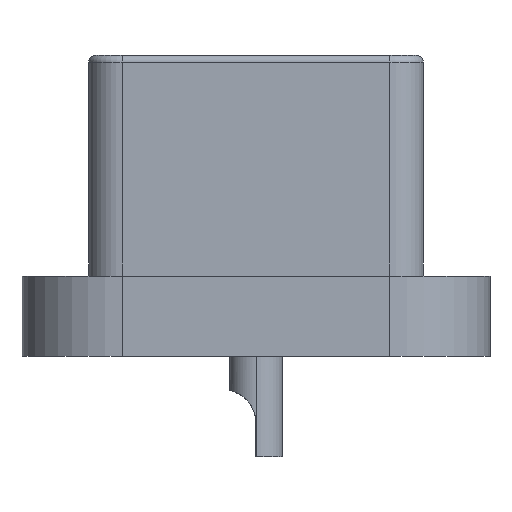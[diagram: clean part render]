
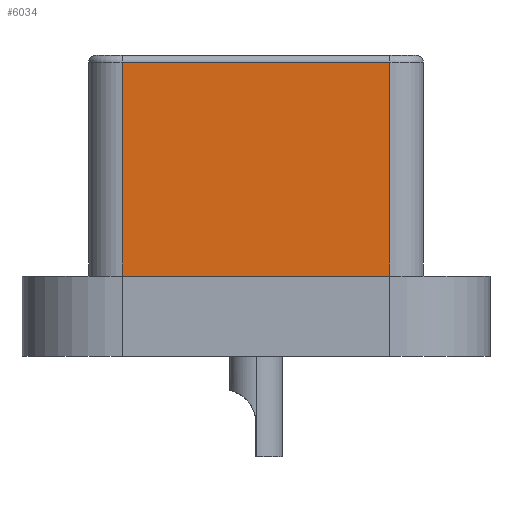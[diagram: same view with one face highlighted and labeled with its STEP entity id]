
A CAD part, left-side view. The second image highlights one B-rep face of the part: STEP entity #6034.
In plain terms, the highlighted planar face has unit normal (-1, 0, 0).
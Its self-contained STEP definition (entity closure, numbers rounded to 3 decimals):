
#138 = ORIENTED_EDGE ( 'NONE', *, *, #6777, .T. ) ;
#802 = CARTESIAN_POINT ( 'NONE',  ( -9.65, -2., -3.3 ) ) ;
#961 = CARTESIAN_POINT ( 'NONE',  ( -9.65, 2., -3.3 ) ) ;
#1038 = DIRECTION ( 'NONE',  ( 0., 0., 1. ) ) ;
#1073 = CARTESIAN_POINT ( 'NONE',  ( -9.65, 2., -3.3 ) ) ;
#1573 = LINE ( 'NONE', #4116, #3683 ) ;
#1833 = VECTOR ( 'NONE', #7389, 1000. ) ;
#1852 = DIRECTION ( 'NONE',  ( 0., 1., 0. ) ) ;
#1875 = VECTOR ( 'NONE', #3530, 1000. ) ;
#1914 = VERTEX_POINT ( 'NONE', #802 ) ;
#2334 = LINE ( 'NONE', #4892, #1833 ) ;
#2479 = PLANE ( 'NONE',  #5477 ) ;
#2680 = EDGE_LOOP ( 'NONE', ( #7239, #3407, #2872, #138 ) ) ;
#2872 = ORIENTED_EDGE ( 'NONE', *, *, #5571, .T. ) ;
#3407 = ORIENTED_EDGE ( 'NONE', *, *, #5192, .T. ) ;
#3530 = DIRECTION ( 'NONE',  ( 0., -1., 0. ) ) ;
#3683 = VECTOR ( 'NONE', #6683, 1000. ) ;
#3967 = VECTOR ( 'NONE', #1038, 1000. ) ;
#4116 = CARTESIAN_POINT ( 'NONE',  ( -9.65, 2., -0.1 ) ) ;
#4228 = LINE ( 'NONE', #6780, #3967 ) ;
#4729 = VERTEX_POINT ( 'NONE', #1073 ) ;
#4892 = CARTESIAN_POINT ( 'NONE',  ( -9.65, -2., -0.1 ) ) ;
#5035 = CARTESIAN_POINT ( 'NONE',  ( -9.65, 0., -1.7 ) ) ;
#5192 = EDGE_CURVE ( 'NONE', #4729, #1914, #6718, .T. ) ;
#5477 = AXIS2_PLACEMENT_3D ( 'NONE', #5035, #7516, #1852 ) ;
#5571 = EDGE_CURVE ( 'NONE', #1914, #7603, #4228, .T. ) ;
#6034 = ADVANCED_FACE ( 'NONE', ( #8121 ), #2479, .F. ) ;
#6237 = CARTESIAN_POINT ( 'NONE',  ( -9.65, -2., -0.1 ) ) ;
#6532 = CARTESIAN_POINT ( 'NONE',  ( -9.65, 2., -0.1 ) ) ;
#6683 = DIRECTION ( 'NONE',  ( 0., 0., -1. ) ) ;
#6688 = EDGE_CURVE ( 'NONE', #7359, #4729, #1573, .T. ) ;
#6718 = LINE ( 'NONE', #961, #1875 ) ;
#6777 = EDGE_CURVE ( 'NONE', #7603, #7359, #2334, .T. ) ;
#6780 = CARTESIAN_POINT ( 'NONE',  ( -9.65, -2., -3.3 ) ) ;
#7239 = ORIENTED_EDGE ( 'NONE', *, *, #6688, .T. ) ;
#7359 = VERTEX_POINT ( 'NONE', #6532 ) ;
#7389 = DIRECTION ( 'NONE',  ( 0., 1., 0. ) ) ;
#7516 = DIRECTION ( 'NONE',  ( 1., 0., 0. ) ) ;
#7603 = VERTEX_POINT ( 'NONE', #6237 ) ;
#8121 = FACE_OUTER_BOUND ( 'NONE', #2680, .T. ) ;
